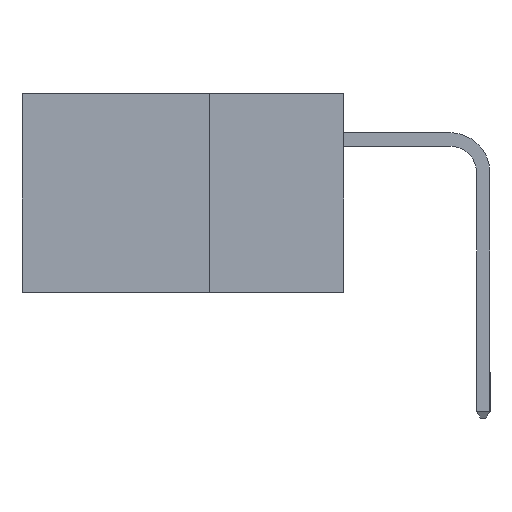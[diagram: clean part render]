
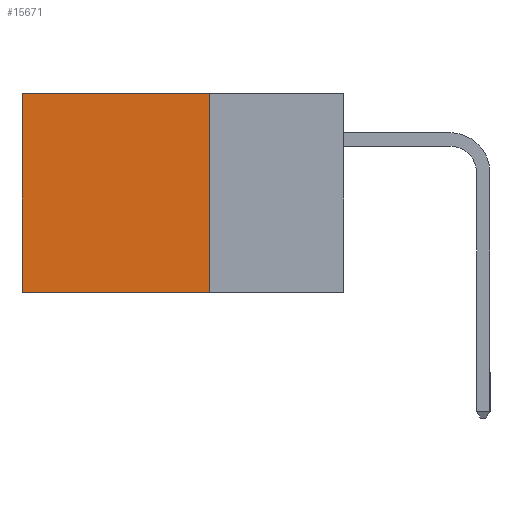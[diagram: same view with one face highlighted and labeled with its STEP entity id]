
A CAD part, left-side view. The second image highlights one B-rep face of the part: STEP entity #15671.
In plain terms, the highlighted planar face has unit normal (-1, 0, 0).
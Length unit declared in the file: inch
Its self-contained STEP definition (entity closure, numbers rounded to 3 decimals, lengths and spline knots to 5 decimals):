
#293 = DIRECTION ( 'NONE',  ( 0., 1., 0. ) ) ;
#494 = LINE ( 'NONE', #18620, #17626 ) ;
#918 = DIRECTION ( 'NONE',  ( 1., 0., 0. ) ) ;
#1823 = CARTESIAN_POINT ( 'NONE',  ( 0.298, 0.25, -0.37 ) ) ;
#2011 = VERTEX_POINT ( 'NONE', #4932 ) ;
#2222 = CARTESIAN_POINT ( 'NONE',  ( 0.298, 0.25, 0. ) ) ;
#3469 = DIRECTION ( 'NONE',  ( 0., 1., 0. ) ) ;
#4302 = CARTESIAN_POINT ( 'NONE',  ( 0.298, 0.25, 0. ) ) ;
#4576 = CARTESIAN_POINT ( 'NONE',  ( 0.298, 0.6, 0. ) ) ;
#4932 = CARTESIAN_POINT ( 'NONE',  ( 0.298, 0.6, -0.37 ) ) ;
#5344 = VECTOR ( 'NONE', #16869, 39.37008 ) ;
#6205 = VECTOR ( 'NONE', #15625, 39.37008 ) ;
#7551 = AXIS2_PLACEMENT_3D ( 'NONE', #4302, #918, #19343 ) ;
#8253 = VECTOR ( 'NONE', #293, 39.37008 ) ;
#9272 = CARTESIAN_POINT ( 'NONE',  ( 0.298, 0.25, 0. ) ) ;
#10922 = VERTEX_POINT ( 'NONE', #1823 ) ;
#11604 = LINE ( 'NONE', #13782, #5344 ) ;
#11783 = VERTEX_POINT ( 'NONE', #9272 ) ;
#11952 = ORIENTED_EDGE ( 'NONE', *, *, #13497, .T. ) ;
#12139 = EDGE_CURVE ( 'NONE', #11783, #10922, #12713, .T. ) ;
#12671 = LINE ( 'NONE', #18417, #8253 ) ;
#12713 = LINE ( 'NONE', #2222, #6205 ) ;
#13471 = EDGE_CURVE ( 'NONE', #10922, #2011, #494, .T. ) ;
#13497 = EDGE_CURVE ( 'NONE', #11783, #20107, #12671, .T. ) ;
#13782 = CARTESIAN_POINT ( 'NONE',  ( 0.298, 0.6, 0. ) ) ;
#14631 = EDGE_CURVE ( 'NONE', #20107, #2011, #11604, .T. ) ;
#14656 = ORIENTED_EDGE ( 'NONE', *, *, #13471, .F. ) ;
#15625 = DIRECTION ( 'NONE',  ( 0., 0., -1. ) ) ;
#15671 = ADVANCED_FACE ( 'NONE', ( #16766 ), #17472, .F. ) ;
#16766 = FACE_OUTER_BOUND ( 'NONE', #19074, .T. ) ;
#16869 = DIRECTION ( 'NONE',  ( 0., 0., -1. ) ) ;
#17472 = PLANE ( 'NONE',  #7551 ) ;
#17626 = VECTOR ( 'NONE', #3469, 39.37008 ) ;
#17888 = ORIENTED_EDGE ( 'NONE', *, *, #14631, .T. ) ;
#18417 = CARTESIAN_POINT ( 'NONE',  ( 0.298, 0.25, 0. ) ) ;
#18620 = CARTESIAN_POINT ( 'NONE',  ( 0.298, 0.25, -0.37 ) ) ;
#19074 = EDGE_LOOP ( 'NONE', ( #17888, #14656, #19932, #11952 ) ) ;
#19343 = DIRECTION ( 'NONE',  ( 0., 0., -1. ) ) ;
#19932 = ORIENTED_EDGE ( 'NONE', *, *, #12139, .F. ) ;
#20107 = VERTEX_POINT ( 'NONE', #4576 ) ;
